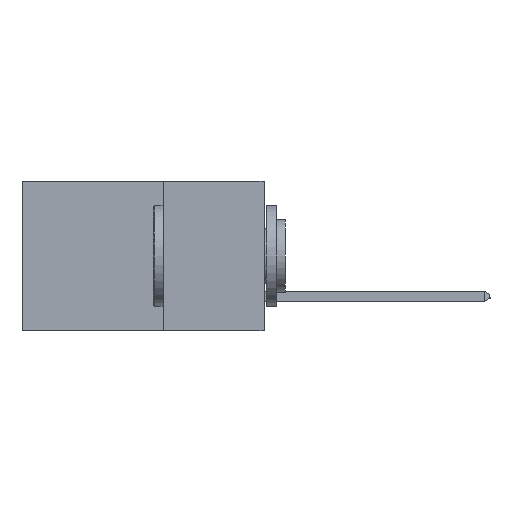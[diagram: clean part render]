
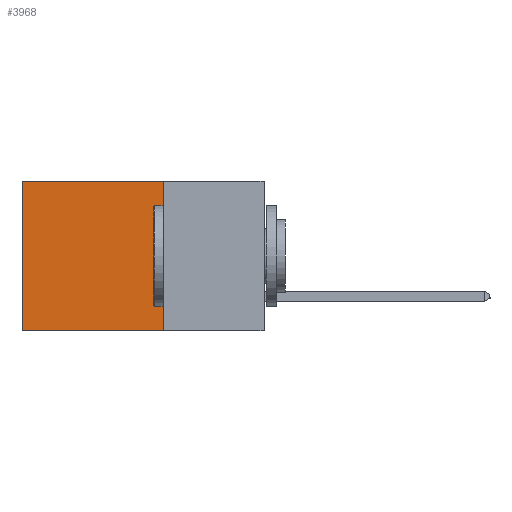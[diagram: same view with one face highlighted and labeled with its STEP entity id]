
A CAD part, left-side view. The second image highlights one B-rep face of the part: STEP entity #3968.
In plain terms, the highlighted planar face has unit normal (-1, 0, 0).
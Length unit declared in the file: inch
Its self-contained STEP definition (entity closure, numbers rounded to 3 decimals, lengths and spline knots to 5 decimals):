
#63 = VECTOR ( 'NONE', #491, 39.37008 ) ;
#98 = VERTEX_POINT ( 'NONE', #16429 ) ;
#350 = ORIENTED_EDGE ( 'NONE', *, *, #17286, .T. ) ;
#386 = CARTESIAN_POINT ( 'NONE',  ( 0.298, 0.25, 0. ) ) ;
#491 = DIRECTION ( 'NONE',  ( 0., 1., 0. ) ) ;
#1064 = VERTEX_POINT ( 'NONE', #14970 ) ;
#1727 = VECTOR ( 'NONE', #13078, 39.37008 ) ;
#2222 = AXIS2_PLACEMENT_3D ( 'NONE', #17627, #18526, #18187 ) ;
#2501 = ORIENTED_EDGE ( 'NONE', *, *, #15103, .F. ) ;
#3014 = LINE ( 'NONE', #10271, #18072 ) ;
#3968 = ADVANCED_FACE ( 'NONE', ( #17833 ), #17506, .F. ) ;
#3989 = ORIENTED_EDGE ( 'NONE', *, *, #9217, .T. ) ;
#4703 = DIRECTION ( 'NONE',  ( 0., 0., -1. ) ) ;
#5832 = LINE ( 'NONE', #8547, #1727 ) ;
#8072 = ORIENTED_EDGE ( 'NONE', *, *, #12112, .F. ) ;
#8547 = CARTESIAN_POINT ( 'NONE',  ( 0.298, 0.6, 0. ) ) ;
#8679 = CARTESIAN_POINT ( 'NONE',  ( 0.298, 0.25, -0.37 ) ) ;
#8717 = LINE ( 'NONE', #386, #63 ) ;
#9217 = EDGE_CURVE ( 'NONE', #1064, #18249, #8717, .T. ) ;
#10001 = LINE ( 'NONE', #16002, #17137 ) ;
#10271 = CARTESIAN_POINT ( 'NONE',  ( 0.298, 0.25, 0. ) ) ;
#12061 = VERTEX_POINT ( 'NONE', #8679 ) ;
#12112 = EDGE_CURVE ( 'NONE', #12061, #98, #10001, .T. ) ;
#13078 = DIRECTION ( 'NONE',  ( 0., 0., -1. ) ) ;
#14056 = CARTESIAN_POINT ( 'NONE',  ( 0.298, 0.6, 0. ) ) ;
#14970 = CARTESIAN_POINT ( 'NONE',  ( 0.298, 0.25, 0. ) ) ;
#15103 = EDGE_CURVE ( 'NONE', #1064, #12061, #3014, .T. ) ;
#16002 = CARTESIAN_POINT ( 'NONE',  ( 0.298, 0.25, -0.37 ) ) ;
#16429 = CARTESIAN_POINT ( 'NONE',  ( 0.298, 0.6, -0.37 ) ) ;
#17137 = VECTOR ( 'NONE', #17352, 39.37008 ) ;
#17286 = EDGE_CURVE ( 'NONE', #18249, #98, #5832, .T. ) ;
#17352 = DIRECTION ( 'NONE',  ( 0., 1., 0. ) ) ;
#17506 = PLANE ( 'NONE',  #2222 ) ;
#17627 = CARTESIAN_POINT ( 'NONE',  ( 0.298, 0.25, 0. ) ) ;
#17833 = FACE_OUTER_BOUND ( 'NONE', #18427, .T. ) ;
#18072 = VECTOR ( 'NONE', #4703, 39.37008 ) ;
#18187 = DIRECTION ( 'NONE',  ( 0., 0., -1. ) ) ;
#18249 = VERTEX_POINT ( 'NONE', #14056 ) ;
#18427 = EDGE_LOOP ( 'NONE', ( #350, #8072, #2501, #3989 ) ) ;
#18526 = DIRECTION ( 'NONE',  ( 1., 0., 0. ) ) ;
